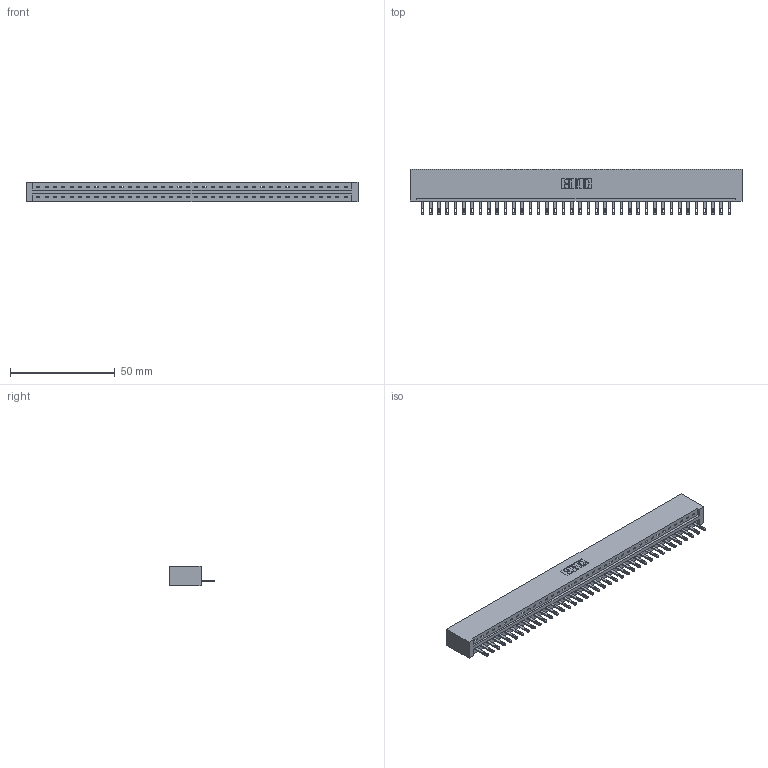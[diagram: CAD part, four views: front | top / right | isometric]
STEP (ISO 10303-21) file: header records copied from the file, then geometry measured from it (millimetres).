
FILE_DESCRIPTION (( 'STEP AP203' ), '1' );
FILE_NAME ('337-038-500-101.STEP', '2019-10-01T16:14:31', ( '' ), ( '' ), 'SwSTEP 2.0', 'SolidWorks 2016', '' );
FILE_SCHEMA (( 'CONFIG_CONTROL_DESIGN' ));
Length unit declared in the file: inch
Products named in the file (3): 345-292-001_345-293-100; 337-038-500-101; 337 Part_No Mounting Lugs
Assembly tree (39 placements, depth 2):
  337-038-500-101
    337 Part_No Mounting Lugs
    345-292-001_345-293-100  x38
Bounding box: 158.45 x 21.85 x 9.4 mm (x, y, z)
Volume: 17179.9 mm3; surface area: 17800.8 mm2
Topology: 39 solids, 39 shells, 2310 faces, 7127 edges, 4750 vertices
Faces by surface type: plane 1586, cylinder 724
Entity records: 28417 total; most frequent: CARTESIAN_POINT 4956, ORIENTED_EDGE 4930, DIRECTION 4173, EDGE_CURVE 2465, LINE 2341, VECTOR 2341, VERTEX_POINT 1642, AXIS2_PLACEMENT_3D 916
